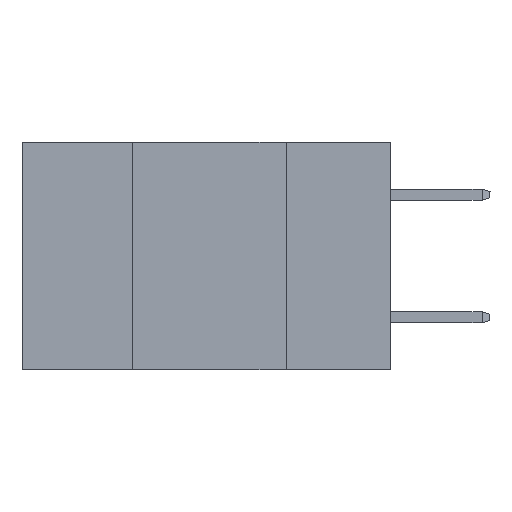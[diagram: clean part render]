
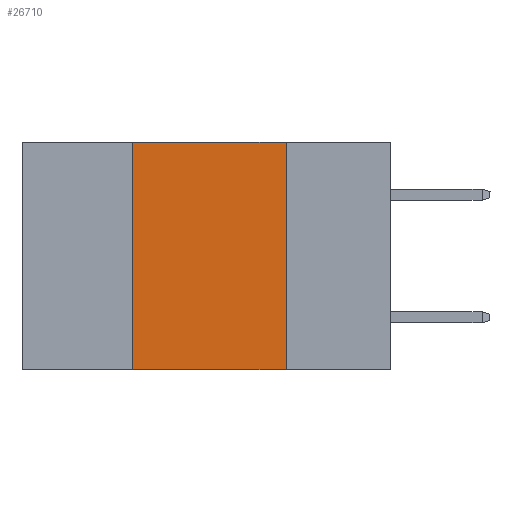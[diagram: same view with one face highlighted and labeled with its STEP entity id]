
A CAD part, left-side view. The second image highlights one B-rep face of the part: STEP entity #26710.
In plain terms, the highlighted planar face has unit normal (-1, 0, 0).
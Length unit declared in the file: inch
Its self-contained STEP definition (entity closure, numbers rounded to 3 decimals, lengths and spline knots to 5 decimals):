
#1605 = CARTESIAN_POINT ( 'NONE',  ( 0., 0.42, -0.37 ) ) ;
#3200 = CARTESIAN_POINT ( 'NONE',  ( 0., 0.6, 0. ) ) ;
#3491 = LINE ( 'NONE', #3200, #13484 ) ;
#3698 = PLANE ( 'NONE',  #13235 ) ;
#7479 = DIRECTION ( 'NONE',  ( 0., -1., 0. ) ) ;
#7665 = DIRECTION ( 'NONE',  ( 0., -1., 0. ) ) ;
#8815 = ORIENTED_EDGE ( 'NONE', *, *, #9009, .T. ) ;
#9009 = EDGE_CURVE ( 'NONE', #16502, #13596, #13805, .T. ) ;
#9896 = DIRECTION ( 'NONE',  ( 1., 0., 0. ) ) ;
#11566 = VECTOR ( 'NONE', #18440, 39.37008 ) ;
#11875 = ORIENTED_EDGE ( 'NONE', *, *, #17585, .F. ) ;
#12160 = CARTESIAN_POINT ( 'NONE',  ( 0., 0.17, 0. ) ) ;
#12169 = VECTOR ( 'NONE', #7479, 39.37008 ) ;
#13235 = AXIS2_PLACEMENT_3D ( 'NONE', #18667, #9896, #25410 ) ;
#13484 = VECTOR ( 'NONE', #7665, 39.37008 ) ;
#13596 = VERTEX_POINT ( 'NONE', #16029 ) ;
#13805 = LINE ( 'NONE', #25140, #12169 ) ;
#14269 = CARTESIAN_POINT ( 'NONE',  ( 0., 0.42, 0. ) ) ;
#14930 = CARTESIAN_POINT ( 'NONE',  ( 0., 0.17, 0. ) ) ;
#15639 = EDGE_LOOP ( 'NONE', ( #21120, #27637, #11875, #8815 ) ) ;
#16029 = CARTESIAN_POINT ( 'NONE',  ( 0., 0.17, -0.37 ) ) ;
#16502 = VERTEX_POINT ( 'NONE', #1605 ) ;
#16573 = CARTESIAN_POINT ( 'NONE',  ( 0., 0.42, 0. ) ) ;
#16746 = LINE ( 'NONE', #12160, #22541 ) ;
#17190 = EDGE_CURVE ( 'NONE', #20198, #13596, #16746, .T. ) ;
#17585 = EDGE_CURVE ( 'NONE', #16502, #23359, #27477, .T. ) ;
#18440 = DIRECTION ( 'NONE',  ( 0., 0., 1. ) ) ;
#18667 = CARTESIAN_POINT ( 'NONE',  ( 0., 0.6, 0. ) ) ;
#20198 = VERTEX_POINT ( 'NONE', #14930 ) ;
#20995 = EDGE_CURVE ( 'NONE', #23359, #20198, #3491, .T. ) ;
#21120 = ORIENTED_EDGE ( 'NONE', *, *, #17190, .F. ) ;
#21381 = FACE_OUTER_BOUND ( 'NONE', #15639, .T. ) ;
#22541 = VECTOR ( 'NONE', #25206, 39.37008 ) ;
#23359 = VERTEX_POINT ( 'NONE', #16573 ) ;
#25140 = CARTESIAN_POINT ( 'NONE',  ( 0., 0.6, -0.37 ) ) ;
#25206 = DIRECTION ( 'NONE',  ( 0., 0., -1. ) ) ;
#25410 = DIRECTION ( 'NONE',  ( 0., 0., -1. ) ) ;
#26710 = ADVANCED_FACE ( 'NONE', ( #21381 ), #3698, .F. ) ;
#27477 = LINE ( 'NONE', #14269, #11566 ) ;
#27637 = ORIENTED_EDGE ( 'NONE', *, *, #20995, .F. ) ;
